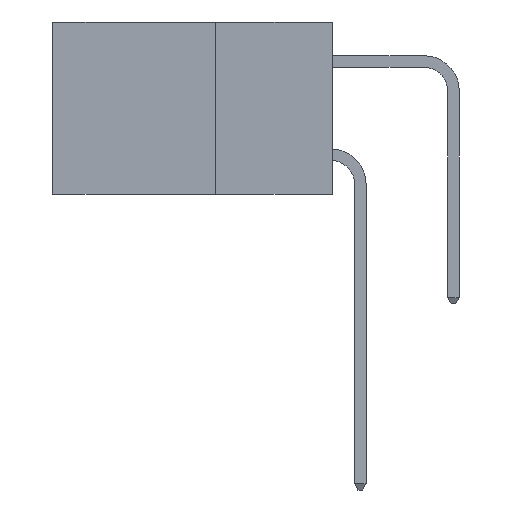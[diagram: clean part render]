
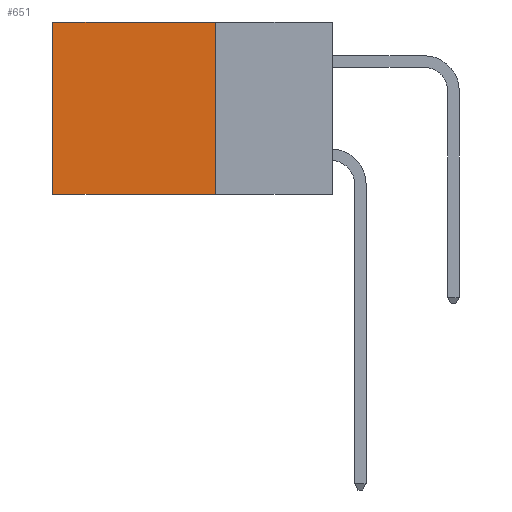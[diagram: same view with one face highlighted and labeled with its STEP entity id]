
A CAD part, left-side view. The second image highlights one B-rep face of the part: STEP entity #651.
In plain terms, the highlighted planar face has unit normal (-1, 0, 0).
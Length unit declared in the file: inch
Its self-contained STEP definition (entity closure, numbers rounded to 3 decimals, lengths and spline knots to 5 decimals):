
#40 = VERTEX_POINT ( 'NONE', #16219 ) ;
#134 = LINE ( 'NONE', #13657, #15516 ) ;
#651 = ADVANCED_FACE ( 'NONE', ( #8842 ), #13084, .F. ) ;
#1899 = VERTEX_POINT ( 'NONE', #16788 ) ;
#2697 = CARTESIAN_POINT ( 'NONE',  ( 0.2615, 0.6, -0.37 ) ) ;
#2833 = VECTOR ( 'NONE', #5855, 39.37008 ) ;
#3356 = CARTESIAN_POINT ( 'NONE',  ( 0.2615, 0.25, 0. ) ) ;
#5855 = DIRECTION ( 'NONE',  ( 0., 1., 0. ) ) ;
#5987 = EDGE_CURVE ( 'NONE', #18166, #40, #13375, .T. ) ;
#6932 = LINE ( 'NONE', #15925, #2833 ) ;
#7759 = ORIENTED_EDGE ( 'NONE', *, *, #18346, .T. ) ;
#8110 = DIRECTION ( 'NONE',  ( 0., 1., 0. ) ) ;
#8255 = CARTESIAN_POINT ( 'NONE',  ( 0.2615, 0.25, 0. ) ) ;
#8659 = DIRECTION ( 'NONE',  ( 0., 0., -1. ) ) ;
#8735 = CARTESIAN_POINT ( 'NONE',  ( 0.2615, 0.25, -0.37 ) ) ;
#8842 = FACE_OUTER_BOUND ( 'NONE', #16975, .T. ) ;
#8998 = AXIS2_PLACEMENT_3D ( 'NONE', #8735, #11947, #8659 ) ;
#9406 = DIRECTION ( 'NONE',  ( 0., 0., -1. ) ) ;
#9586 = VECTOR ( 'NONE', #8110, 39.37008 ) ;
#9635 = ORIENTED_EDGE ( 'NONE', *, *, #16858, .F. ) ;
#9937 = CARTESIAN_POINT ( 'NONE',  ( 0.2615, 0.6, -0.37 ) ) ;
#11376 = DIRECTION ( 'NONE',  ( 0., 0., -1. ) ) ;
#11715 = LINE ( 'NONE', #9937, #18738 ) ;
#11836 = EDGE_CURVE ( 'NONE', #1899, #18510, #6932, .T. ) ;
#11947 = DIRECTION ( 'NONE',  ( 1., 0., 0. ) ) ;
#13084 = PLANE ( 'NONE',  #8998 ) ;
#13375 = LINE ( 'NONE', #8255, #9586 ) ;
#13657 = CARTESIAN_POINT ( 'NONE',  ( 0.2615, 0.25, -0.37 ) ) ;
#15516 = VECTOR ( 'NONE', #9406, 39.37008 ) ;
#15925 = CARTESIAN_POINT ( 'NONE',  ( 0.2615, 0.25, -0.37 ) ) ;
#16219 = CARTESIAN_POINT ( 'NONE',  ( 0.2615, 0.6, 0. ) ) ;
#16268 = ORIENTED_EDGE ( 'NONE', *, *, #11836, .F. ) ;
#16505 = ORIENTED_EDGE ( 'NONE', *, *, #5987, .T. ) ;
#16788 = CARTESIAN_POINT ( 'NONE',  ( 0.2615, 0.25, -0.37 ) ) ;
#16858 = EDGE_CURVE ( 'NONE', #18166, #1899, #134, .T. ) ;
#16975 = EDGE_LOOP ( 'NONE', ( #7759, #16268, #9635, #16505 ) ) ;
#18166 = VERTEX_POINT ( 'NONE', #3356 ) ;
#18346 = EDGE_CURVE ( 'NONE', #40, #18510, #11715, .T. ) ;
#18510 = VERTEX_POINT ( 'NONE', #2697 ) ;
#18738 = VECTOR ( 'NONE', #11376, 39.37008 ) ;
